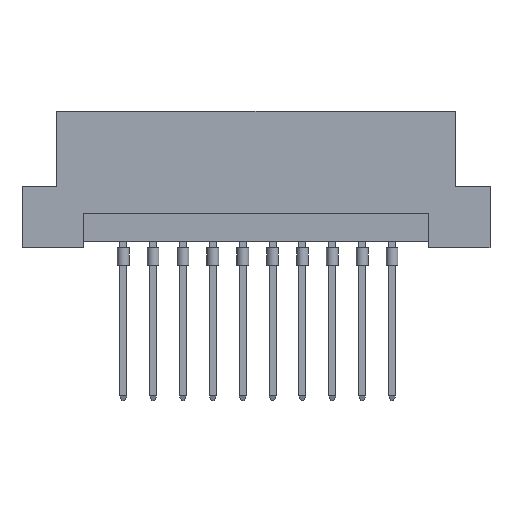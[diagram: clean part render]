
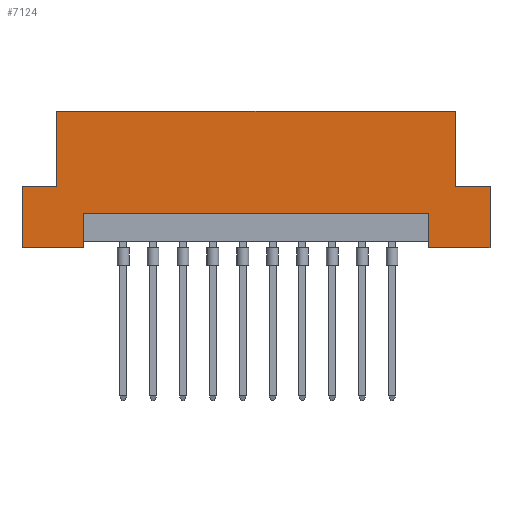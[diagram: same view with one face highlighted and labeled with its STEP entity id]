
A CAD part, front view. The second image highlights one B-rep face of the part: STEP entity #7124.
In plain terms, the highlighted planar face has unit normal (0, -1, 0).
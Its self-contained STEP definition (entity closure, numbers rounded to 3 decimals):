
#189 = PLANE ( 'NONE',  #6455 ) ;
#230 = VECTOR ( 'NONE', #5826, 1000. ) ;
#257 = VERTEX_POINT ( 'NONE', #941 ) ;
#272 = VERTEX_POINT ( 'NONE', #7408 ) ;
#436 = VERTEX_POINT ( 'NONE', #3418 ) ;
#589 = VERTEX_POINT ( 'NONE', #1896 ) ;
#661 = EDGE_CURVE ( 'NONE', #880, #2723, #3639, .T. ) ;
#866 = LINE ( 'NONE', #7368, #2639 ) ;
#880 = VERTEX_POINT ( 'NONE', #5103 ) ;
#941 = CARTESIAN_POINT ( 'NONE',  ( -16.94, 0., 5.2 ) ) ;
#1069 = VECTOR ( 'NONE', #1717, 1000. ) ;
#1095 = ORIENTED_EDGE ( 'NONE', *, *, #1974, .F. ) ;
#1136 = VECTOR ( 'NONE', #2835, 1000. ) ;
#1186 = LINE ( 'NONE', #2913, #1237 ) ;
#1230 = CARTESIAN_POINT ( 'NONE',  ( 16.94, 0., 5.2 ) ) ;
#1237 = VECTOR ( 'NONE', #7072, 1000. ) ;
#1476 = DIRECTION ( 'NONE',  ( 0., 0., 1. ) ) ;
#1568 = VECTOR ( 'NONE', #2365, 1000. ) ;
#1682 = EDGE_CURVE ( 'NONE', #7203, #5464, #1814, .T. ) ;
#1717 = DIRECTION ( 'NONE',  ( 1., 0., 0. ) ) ;
#1748 = LINE ( 'NONE', #5269, #230 ) ;
#1814 = LINE ( 'NONE', #7082, #7131 ) ;
#1863 = VERTEX_POINT ( 'NONE', #1890 ) ;
#1865 = DIRECTION ( 'NONE',  ( 1., 0., 0. ) ) ;
#1890 = CARTESIAN_POINT ( 'NONE',  ( -19.9, 0., 0. ) ) ;
#1896 = CARTESIAN_POINT ( 'NONE',  ( 19.9, 0., 5.2 ) ) ;
#1909 = CARTESIAN_POINT ( 'NONE',  ( -19.9, 0., 11.6 ) ) ;
#1974 = EDGE_CURVE ( 'NONE', #589, #7203, #6228, .T. ) ;
#2047 = VECTOR ( 'NONE', #3368, 1000. ) ;
#2081 = DIRECTION ( 'NONE',  ( 0., 0., -1. ) ) ;
#2168 = EDGE_CURVE ( 'NONE', #6840, #880, #1186, .T. ) ;
#2199 = CARTESIAN_POINT ( 'NONE',  ( -19.9, 0., 0. ) ) ;
#2200 = DIRECTION ( 'NONE',  ( 1., 0., 0. ) ) ;
#2205 = ORIENTED_EDGE ( 'NONE', *, *, #3264, .F. ) ;
#2216 = ORIENTED_EDGE ( 'NONE', *, *, #5503, .F. ) ;
#2365 = DIRECTION ( 'NONE',  ( 0., 0., 1. ) ) ;
#2400 = CARTESIAN_POINT ( 'NONE',  ( -16.94, 0., 11.6 ) ) ;
#2639 = VECTOR ( 'NONE', #6127, 1000. ) ;
#2723 = VERTEX_POINT ( 'NONE', #7103 ) ;
#2835 = DIRECTION ( 'NONE',  ( 0., 0., -1. ) ) ;
#2913 = CARTESIAN_POINT ( 'NONE',  ( 14.69, 0., 2.9 ) ) ;
#3032 = DIRECTION ( 'NONE',  ( 0., 0., -1. ) ) ;
#3068 = CARTESIAN_POINT ( 'NONE',  ( -14.69, 0., 0.5 ) ) ;
#3151 = EDGE_CURVE ( 'NONE', #257, #7418, #1748, .T. ) ;
#3264 = EDGE_CURVE ( 'NONE', #272, #257, #4761, .T. ) ;
#3308 = CARTESIAN_POINT ( 'NONE',  ( 19.9, 0., 0. ) ) ;
#3368 = DIRECTION ( 'NONE',  ( 0., 0., 1. ) ) ;
#3406 = LINE ( 'NONE', #3984, #4500 ) ;
#3418 = CARTESIAN_POINT ( 'NONE',  ( 16.94, 0., 11.6 ) ) ;
#3508 = LINE ( 'NONE', #4129, #1568 ) ;
#3509 = CARTESIAN_POINT ( 'NONE',  ( 19.9, 0., 5.2 ) ) ;
#3639 = LINE ( 'NONE', #3068, #4677 ) ;
#3746 = ORIENTED_EDGE ( 'NONE', *, *, #3151, .F. ) ;
#3887 = EDGE_CURVE ( 'NONE', #6531, #436, #3508, .T. ) ;
#3984 = CARTESIAN_POINT ( 'NONE',  ( -19.9, 0., 11.6 ) ) ;
#4129 = CARTESIAN_POINT ( 'NONE',  ( 16.94, 0., 5.2 ) ) ;
#4212 = EDGE_CURVE ( 'NONE', #2723, #1863, #866, .T. ) ;
#4229 = EDGE_LOOP ( 'NONE', ( #6718, #6642, #7286, #1095, #2216, #6571, #5053, #3746, #2205, #7142, #5169, #4848 ) ) ;
#4326 = LINE ( 'NONE', #7311, #5454 ) ;
#4500 = VECTOR ( 'NONE', #2200, 1000. ) ;
#4540 = CARTESIAN_POINT ( 'NONE',  ( 14.69, 0., 2.9 ) ) ;
#4677 = VECTOR ( 'NONE', #3032, 1000. ) ;
#4761 = LINE ( 'NONE', #7093, #6552 ) ;
#4766 = EDGE_CURVE ( 'NONE', #6840, #5464, #4326, .T. ) ;
#4846 = EDGE_CURVE ( 'NONE', #1863, #272, #4934, .T. ) ;
#4848 = ORIENTED_EDGE ( 'NONE', *, *, #661, .F. ) ;
#4934 = LINE ( 'NONE', #2199, #2047 ) ;
#5053 = ORIENTED_EDGE ( 'NONE', *, *, #6345, .F. ) ;
#5060 = CARTESIAN_POINT ( 'NONE',  ( 19.9, 0., 0. ) ) ;
#5103 = CARTESIAN_POINT ( 'NONE',  ( -14.69, 0., 2.9 ) ) ;
#5169 = ORIENTED_EDGE ( 'NONE', *, *, #4212, .F. ) ;
#5269 = CARTESIAN_POINT ( 'NONE',  ( -16.94, 0., 5.2 ) ) ;
#5292 = DIRECTION ( 'NONE',  ( -1., 0., 0. ) ) ;
#5454 = VECTOR ( 'NONE', #2081, 1000. ) ;
#5464 = VERTEX_POINT ( 'NONE', #5571 ) ;
#5488 = FACE_OUTER_BOUND ( 'NONE', #4229, .T. ) ;
#5503 = EDGE_CURVE ( 'NONE', #6531, #589, #7065, .T. ) ;
#5571 = CARTESIAN_POINT ( 'NONE',  ( 14.69, 0., 0. ) ) ;
#5826 = DIRECTION ( 'NONE',  ( 0., 0., 1. ) ) ;
#6127 = DIRECTION ( 'NONE',  ( -1., 0., 0. ) ) ;
#6228 = LINE ( 'NONE', #5060, #1136 ) ;
#6345 = EDGE_CURVE ( 'NONE', #7418, #436, #3406, .T. ) ;
#6455 = AXIS2_PLACEMENT_3D ( 'NONE', #1909, #7248, #1476 ) ;
#6531 = VERTEX_POINT ( 'NONE', #1230 ) ;
#6552 = VECTOR ( 'NONE', #1865, 1000. ) ;
#6571 = ORIENTED_EDGE ( 'NONE', *, *, #3887, .T. ) ;
#6642 = ORIENTED_EDGE ( 'NONE', *, *, #4766, .T. ) ;
#6718 = ORIENTED_EDGE ( 'NONE', *, *, #2168, .F. ) ;
#6840 = VERTEX_POINT ( 'NONE', #4540 ) ;
#7065 = LINE ( 'NONE', #3509, #1069 ) ;
#7072 = DIRECTION ( 'NONE',  ( -1., 0., 0. ) ) ;
#7082 = CARTESIAN_POINT ( 'NONE',  ( -19.9, 0., 0. ) ) ;
#7093 = CARTESIAN_POINT ( 'NONE',  ( -19.9, 0., 5.2 ) ) ;
#7103 = CARTESIAN_POINT ( 'NONE',  ( -14.69, 0., 0. ) ) ;
#7124 = ADVANCED_FACE ( 'NONE', ( #5488 ), #189, .F. ) ;
#7131 = VECTOR ( 'NONE', #5292, 1000. ) ;
#7142 = ORIENTED_EDGE ( 'NONE', *, *, #4846, .F. ) ;
#7203 = VERTEX_POINT ( 'NONE', #3308 ) ;
#7248 = DIRECTION ( 'NONE',  ( 0., 1., 0. ) ) ;
#7286 = ORIENTED_EDGE ( 'NONE', *, *, #1682, .F. ) ;
#7311 = CARTESIAN_POINT ( 'NONE',  ( 14.69, 0., 0.5 ) ) ;
#7368 = CARTESIAN_POINT ( 'NONE',  ( -19.9, 0., 0. ) ) ;
#7408 = CARTESIAN_POINT ( 'NONE',  ( -19.9, 0., 5.2 ) ) ;
#7418 = VERTEX_POINT ( 'NONE', #2400 ) ;
